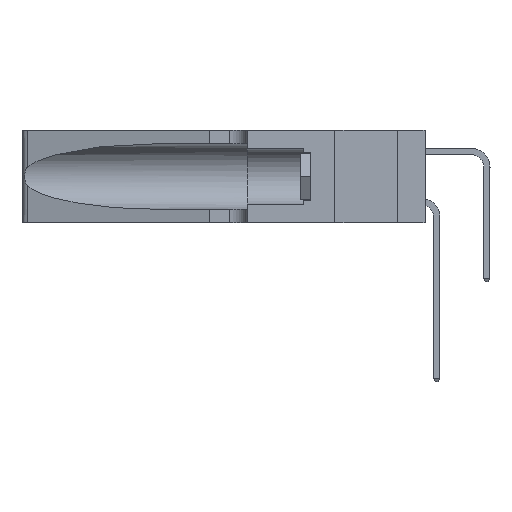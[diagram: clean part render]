
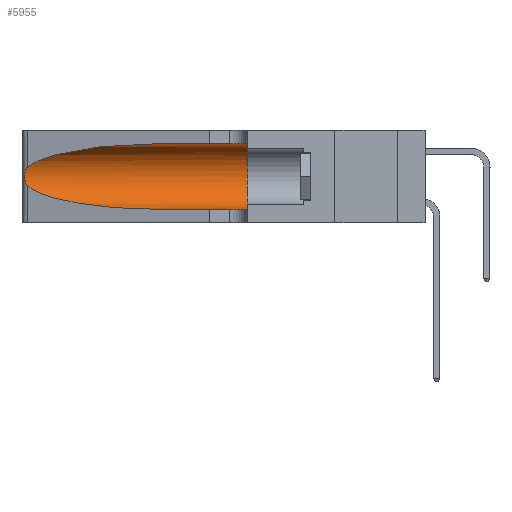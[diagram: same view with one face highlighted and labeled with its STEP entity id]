
A CAD part, left-side view. The second image highlights one B-rep face of the part: STEP entity #5955.
In plain terms, the highlighted cylindrical face has radius 3.308 mm (diameter 6.617 mm), a partial arc.
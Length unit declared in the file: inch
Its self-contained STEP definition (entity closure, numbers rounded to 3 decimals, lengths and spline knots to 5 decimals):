
#407 = CARTESIAN_POINT ( 'NONE',  ( 0.25789, 1.23486, 0.15765 ) ) ;
#412 = VECTOR ( 'NONE', #23865, 39.37008 ) ;
#1342 = CIRCLE ( 'NONE', #5698, 0.13025 ) ;
#1419 = DIRECTION ( 'NONE',  ( 0., 1., 0. ) ) ;
#1926 = VERTEX_POINT ( 'NONE', #6321 ) ;
#2091 = ORIENTED_EDGE ( 'NONE', *, *, #10878, .F. ) ;
#2318 =( BOUNDED_CURVE ( )  B_SPLINE_CURVE ( 3, ( #3283, #12688, #24248, #7148 ),
 .UNSPECIFIED., .F., .F. ) 
 B_SPLINE_CURVE_WITH_KNOTS ( ( 4, 4 ),
 ( 1.5708, 2.84003 ),
 .UNSPECIFIED. ) 
 CURVE ( )  GEOMETRIC_REPRESENTATION_ITEM ( )  RATIONAL_B_SPLINE_CURVE ( ( 1., 0.87, 0.87, 1. ) ) 
 REPRESENTATION_ITEM ( '' )  );
#2706 = CARTESIAN_POINT ( 'NONE',  ( 0.1305, 1.61858, 0.31525 ) ) ;
#3283 = CARTESIAN_POINT ( 'NONE',  ( 0.1305, 0.72297, 0.31525 ) ) ;
#3555 =( BOUNDED_CURVE ( )  B_SPLINE_CURVE ( 3, ( #5995, #19352, #23418, #17652 ),
 .UNSPECIFIED., .F., .F. ) 
 B_SPLINE_CURVE_WITH_KNOTS ( ( 4, 4 ),
 ( 3.44316, 4.71239 ),
 .UNSPECIFIED. ) 
 CURVE ( )  GEOMETRIC_REPRESENTATION_ITEM ( )  RATIONAL_B_SPLINE_CURVE ( ( 1., 0.87, 0.87, 1. ) ) 
 REPRESENTATION_ITEM ( '' )  );
#3623 = ORIENTED_EDGE ( 'NONE', *, *, #24522, .T. ) ;
#4030 = CARTESIAN_POINT ( 'NONE',  ( 0.1305, 1.61858, 0.185 ) ) ;
#4190 = CARTESIAN_POINT ( 'NONE',  ( 0.25555, 1.22994, 0.2215 ) ) ;
#4373 = CARTESIAN_POINT ( 'NONE',  ( 0.25555, 1.22993, 0.14849 ) ) ;
#4434 = CARTESIAN_POINT ( 'NONE',  ( 0.1305, 1.61858, 0.05475 ) ) ;
#4459 = CARTESIAN_POINT ( 'NONE',  ( 0.26075, 1.23896, 0.19203 ) ) ;
#4525 = CARTESIAN_POINT ( 'NONE',  ( 0.1305, 0.72297, 0.31525 ) ) ;
#4561 = VERTEX_POINT ( 'NONE', #19045 ) ;
#5698 = AXIS2_PLACEMENT_3D ( 'NONE', #12748, #1419, #20227 ) ;
#5955 = ADVANCED_FACE ( 'NONE', ( #12203 ), #6319, .F. ) ;
#5995 = CARTESIAN_POINT ( 'NONE',  ( 0.25487, 1.22718, 0.14631 ) ) ;
#6292 = CARTESIAN_POINT ( 'NONE',  ( 0.25487, 1.22718, 0.14631 ) ) ;
#6319 = CYLINDRICAL_SURFACE ( 'NONE', #14939, 0.13025 ) ;
#6321 = CARTESIAN_POINT ( 'NONE',  ( 0.25487, 1.22718, 0.22369 ) ) ;
#6406 = DIRECTION ( 'NONE',  ( 0., -1., 0. ) ) ;
#6877 = ORIENTED_EDGE ( 'NONE', *, *, #18572, .T. ) ;
#7148 = CARTESIAN_POINT ( 'NONE',  ( 0.25487, 1.22718, 0.22369 ) ) ;
#9380 = LINE ( 'NONE', #4434, #412 ) ;
#9904 = CARTESIAN_POINT ( 'NONE',  ( 0.26075, 1.23896, 0.178 ) ) ;
#10153 = CARTESIAN_POINT ( 'NONE',  ( 0.25854, 1.2359, 0.20912 ) ) ;
#10878 = EDGE_CURVE ( 'NONE', #20014, #21876, #1342, .T. ) ;
#11865 = CARTESIAN_POINT ( 'NONE',  ( 0.25639, 1.23186, 0.15144 ) ) ;
#12203 = FACE_OUTER_BOUND ( 'NONE', #17039, .T. ) ;
#12688 = CARTESIAN_POINT ( 'NONE',  ( 0.18966, 0.96281, 0.31525 ) ) ;
#12748 = CARTESIAN_POINT ( 'NONE',  ( 0.1305, 0.35, 0.185 ) ) ;
#12878 = EDGE_CURVE ( 'NONE', #1926, #21185, #17683, .T. ) ;
#13761 = CARTESIAN_POINT ( 'NONE',  ( 0.25856, 1.23593, 0.16098 ) ) ;
#14939 = AXIS2_PLACEMENT_3D ( 'NONE', #4030, #17527, #19153 ) ;
#15178 = ORIENTED_EDGE ( 'NONE', *, *, #16967, .F. ) ;
#15470 = ORIENTED_EDGE ( 'NONE', *, *, #19531, .T. ) ;
#15511 = CARTESIAN_POINT ( 'NONE',  ( 0.25487, 1.22718, 0.22369 ) ) ;
#16967 = EDGE_CURVE ( 'NONE', #24024, #20014, #21891, .T. ) ;
#17039 = EDGE_LOOP ( 'NONE', ( #6877, #21366, #15470, #3623, #2091, #15178 ) ) ;
#17424 = CARTESIAN_POINT ( 'NONE',  ( 0.26018, 1.23835, 0.19895 ) ) ;
#17527 = DIRECTION ( 'NONE',  ( 0., -1., 0. ) ) ;
#17652 = CARTESIAN_POINT ( 'NONE',  ( 0.1305, 0.72297, 0.05475 ) ) ;
#17683 = B_SPLINE_CURVE_WITH_KNOTS ( 'NONE', 3,
 ( #15511, #4190, #21227, #23196, #10153, #17424, #4459, #9904, #23286, #13761, #407, #11865, #4373, #6292 ),
 .UNSPECIFIED., .F., .F.,
 ( 4, 2, 2, 2, 2, 2, 4 ),
 ( 0., 0.00027, 0.00053, 0.00107, 0.0016, 0.00187, 0.00214 ),
 .UNSPECIFIED. ) ;
#18572 = EDGE_CURVE ( 'NONE', #24024, #1926, #2318, .T. ) ;
#19045 = CARTESIAN_POINT ( 'NONE',  ( 0.1305, 0.72297, 0.05475 ) ) ;
#19153 = DIRECTION ( 'NONE',  ( 0., 0., -1. ) ) ;
#19352 = CARTESIAN_POINT ( 'NONE',  ( 0.2373, 1.15595, 0.08982 ) ) ;
#19531 = EDGE_CURVE ( 'NONE', #21185, #4561, #3555, .T. ) ;
#20014 = VERTEX_POINT ( 'NONE', #22513 ) ;
#20091 = VECTOR ( 'NONE', #6406, 39.37008 ) ;
#20227 = DIRECTION ( 'NONE',  ( 0., 0., 1. ) ) ;
#20824 = CARTESIAN_POINT ( 'NONE',  ( 0.25487, 1.22718, 0.14631 ) ) ;
#21185 = VERTEX_POINT ( 'NONE', #20824 ) ;
#21217 = CARTESIAN_POINT ( 'NONE',  ( 0.1305, 0.35, 0.05475 ) ) ;
#21227 = CARTESIAN_POINT ( 'NONE',  ( 0.25639, 1.23184, 0.21858 ) ) ;
#21366 = ORIENTED_EDGE ( 'NONE', *, *, #12878, .T. ) ;
#21876 = VERTEX_POINT ( 'NONE', #21217 ) ;
#21891 = LINE ( 'NONE', #2706, #20091 ) ;
#22513 = CARTESIAN_POINT ( 'NONE',  ( 0.1305, 0.35, 0.31525 ) ) ;
#23196 = CARTESIAN_POINT ( 'NONE',  ( 0.25787, 1.23484, 0.2124 ) ) ;
#23286 = CARTESIAN_POINT ( 'NONE',  ( 0.26017, 1.23833, 0.17102 ) ) ;
#23418 = CARTESIAN_POINT ( 'NONE',  ( 0.18966, 0.96281, 0.05475 ) ) ;
#23865 = DIRECTION ( 'NONE',  ( 0., -1., 0. ) ) ;
#24024 = VERTEX_POINT ( 'NONE', #4525 ) ;
#24248 = CARTESIAN_POINT ( 'NONE',  ( 0.2373, 1.15595, 0.28018 ) ) ;
#24522 = EDGE_CURVE ( 'NONE', #4561, #21876, #9380, .T. ) ;
